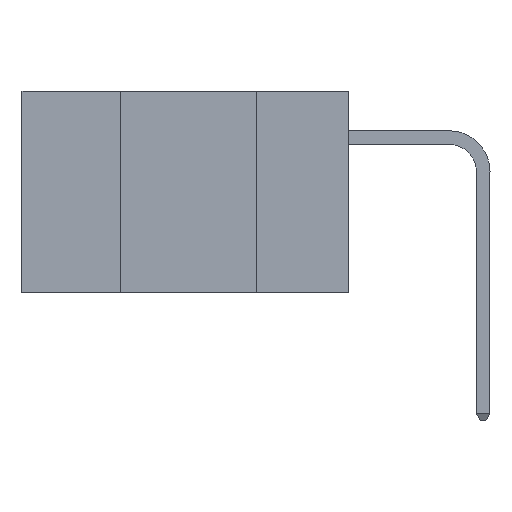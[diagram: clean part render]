
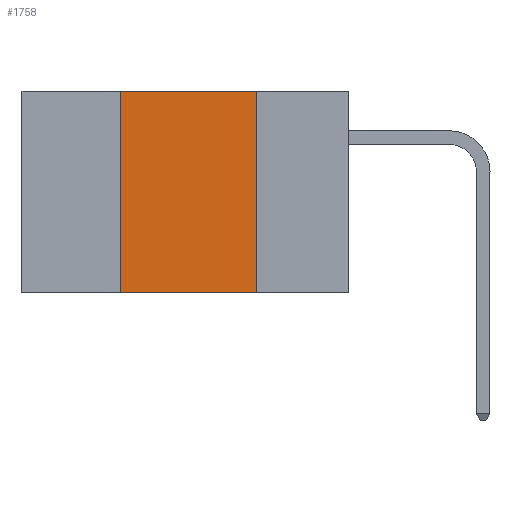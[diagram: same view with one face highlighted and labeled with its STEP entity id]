
A CAD part, left-side view. The second image highlights one B-rep face of the part: STEP entity #1758.
In plain terms, the highlighted planar face has unit normal (-1, 0, 0).
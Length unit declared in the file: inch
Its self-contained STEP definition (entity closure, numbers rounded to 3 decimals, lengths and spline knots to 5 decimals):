
#381 = VECTOR ( 'NONE', #24171, 39.37008 ) ;
#1094 = VECTOR ( 'NONE', #18875, 39.37008 ) ;
#1758 = ADVANCED_FACE ( 'NONE', ( #25189 ), #4510, .F. ) ;
#3488 = ORIENTED_EDGE ( 'NONE', *, *, #8217, .T. ) ;
#4510 = PLANE ( 'NONE',  #16826 ) ;
#5177 = CARTESIAN_POINT ( 'NONE',  ( 0., 0.42, 0. ) ) ;
#7928 = EDGE_CURVE ( 'NONE', #14174, #22066, #24347, .T. ) ;
#8217 = EDGE_CURVE ( 'NONE', #16830, #22066, #10101, .T. ) ;
#8628 = VERTEX_POINT ( 'NONE', #27267 ) ;
#9522 = LINE ( 'NONE', #11536, #20100 ) ;
#10101 = LINE ( 'NONE', #20670, #20693 ) ;
#11536 = CARTESIAN_POINT ( 'NONE',  ( 0., 0.6, 0. ) ) ;
#12912 = CARTESIAN_POINT ( 'NONE',  ( 0., 0.17, -0.37 ) ) ;
#13871 = ORIENTED_EDGE ( 'NONE', *, *, #7928, .F. ) ;
#14174 = VERTEX_POINT ( 'NONE', #25288 ) ;
#14544 = EDGE_LOOP ( 'NONE', ( #13871, #26049, #15688, #3488 ) ) ;
#15688 = ORIENTED_EDGE ( 'NONE', *, *, #26017, .F. ) ;
#16826 = AXIS2_PLACEMENT_3D ( 'NONE', #25394, #23342, #17052 ) ;
#16830 = VERTEX_POINT ( 'NONE', #24921 ) ;
#17052 = DIRECTION ( 'NONE',  ( 0., 0., -1. ) ) ;
#17847 = CARTESIAN_POINT ( 'NONE',  ( 0., 0.17, 0. ) ) ;
#18875 = DIRECTION ( 'NONE',  ( 0., 0., -1. ) ) ;
#19991 = EDGE_CURVE ( 'NONE', #8628, #14174, #9522, .T. ) ;
#20100 = VECTOR ( 'NONE', #24123, 39.37008 ) ;
#20670 = CARTESIAN_POINT ( 'NONE',  ( 0., 0.6, -0.37 ) ) ;
#20693 = VECTOR ( 'NONE', #22786, 39.37008 ) ;
#22066 = VERTEX_POINT ( 'NONE', #12912 ) ;
#22786 = DIRECTION ( 'NONE',  ( 0., -1., 0. ) ) ;
#23286 = LINE ( 'NONE', #5177, #381 ) ;
#23342 = DIRECTION ( 'NONE',  ( 1., 0., 0. ) ) ;
#24123 = DIRECTION ( 'NONE',  ( 0., -1., 0. ) ) ;
#24171 = DIRECTION ( 'NONE',  ( 0., 0., 1. ) ) ;
#24347 = LINE ( 'NONE', #17847, #1094 ) ;
#24921 = CARTESIAN_POINT ( 'NONE',  ( 0., 0.42, -0.37 ) ) ;
#25189 = FACE_OUTER_BOUND ( 'NONE', #14544, .T. ) ;
#25288 = CARTESIAN_POINT ( 'NONE',  ( 0., 0.17, 0. ) ) ;
#25394 = CARTESIAN_POINT ( 'NONE',  ( 0., 0.6, 0. ) ) ;
#26017 = EDGE_CURVE ( 'NONE', #16830, #8628, #23286, .T. ) ;
#26049 = ORIENTED_EDGE ( 'NONE', *, *, #19991, .F. ) ;
#27267 = CARTESIAN_POINT ( 'NONE',  ( 0., 0.42, 0. ) ) ;
